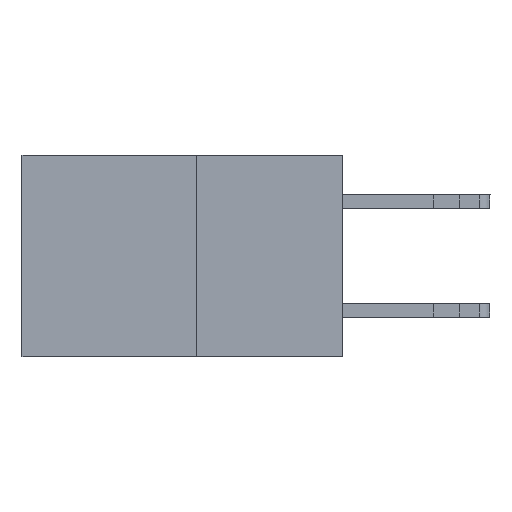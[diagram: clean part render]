
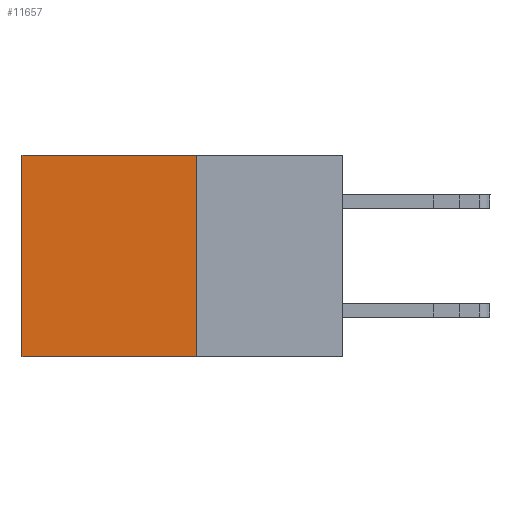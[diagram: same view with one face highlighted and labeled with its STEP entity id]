
A CAD part, left-side view. The second image highlights one B-rep face of the part: STEP entity #11657.
In plain terms, the highlighted planar face has unit normal (-1, 0, 0).
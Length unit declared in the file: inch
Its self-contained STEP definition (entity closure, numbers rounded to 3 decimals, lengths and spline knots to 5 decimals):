
#1325 = DIRECTION ( 'NONE',  ( 1., 0., 0. ) ) ;
#1469 = AXIS2_PLACEMENT_3D ( 'NONE', #7653, #1325, #16634 ) ;
#2169 = VECTOR ( 'NONE', #7233, 39.37008 ) ;
#3443 = CARTESIAN_POINT ( 'NONE',  ( 0.277, 0.27, 0. ) ) ;
#3674 = LINE ( 'NONE', #9184, #3949 ) ;
#3949 = VECTOR ( 'NONE', #5194, 39.37008 ) ;
#4091 = VECTOR ( 'NONE', #10835, 39.37008 ) ;
#5194 = DIRECTION ( 'NONE',  ( 0., 0., -1. ) ) ;
#5997 = CARTESIAN_POINT ( 'NONE',  ( 0.277, 0.59, -0.37 ) ) ;
#6428 = CARTESIAN_POINT ( 'NONE',  ( 0.277, 0.27, 0. ) ) ;
#7233 = DIRECTION ( 'NONE',  ( 0., 1., 0. ) ) ;
#7529 = PLANE ( 'NONE',  #1469 ) ;
#7653 = CARTESIAN_POINT ( 'NONE',  ( 0.277, 0.27, -0.37 ) ) ;
#7782 = FACE_OUTER_BOUND ( 'NONE', #18057, .T. ) ;
#9184 = CARTESIAN_POINT ( 'NONE',  ( 0.277, 0.59, -0.37 ) ) ;
#10682 = EDGE_CURVE ( 'NONE', #21772, #19550, #3674, .T. ) ;
#10835 = DIRECTION ( 'NONE',  ( 0., 1., 0. ) ) ;
#11657 = ADVANCED_FACE ( 'NONE', ( #7782 ), #7529, .F. ) ;
#13093 = ORIENTED_EDGE ( 'NONE', *, *, #20585, .F. ) ;
#15268 = VERTEX_POINT ( 'NONE', #6428 ) ;
#15631 = VECTOR ( 'NONE', #23907, 39.37008 ) ;
#15726 = CARTESIAN_POINT ( 'NONE',  ( 0.277, 0.59, 0. ) ) ;
#16035 = CARTESIAN_POINT ( 'NONE',  ( 0.277, 0.27, -0.37 ) ) ;
#16597 = ORIENTED_EDGE ( 'NONE', *, *, #10682, .T. ) ;
#16634 = DIRECTION ( 'NONE',  ( 0., 0., -1. ) ) ;
#17021 = LINE ( 'NONE', #24538, #2169 ) ;
#18057 = EDGE_LOOP ( 'NONE', ( #16597, #13093, #18802, #19836 ) ) ;
#18802 = ORIENTED_EDGE ( 'NONE', *, *, #23367, .F. ) ;
#19550 = VERTEX_POINT ( 'NONE', #5997 ) ;
#19741 = EDGE_CURVE ( 'NONE', #15268, #21772, #20612, .T. ) ;
#19836 = ORIENTED_EDGE ( 'NONE', *, *, #19741, .T. ) ;
#20003 = LINE ( 'NONE', #23535, #15631 ) ;
#20402 = VERTEX_POINT ( 'NONE', #16035 ) ;
#20585 = EDGE_CURVE ( 'NONE', #20402, #19550, #17021, .T. ) ;
#20612 = LINE ( 'NONE', #3443, #4091 ) ;
#21772 = VERTEX_POINT ( 'NONE', #15726 ) ;
#23367 = EDGE_CURVE ( 'NONE', #15268, #20402, #20003, .T. ) ;
#23535 = CARTESIAN_POINT ( 'NONE',  ( 0.277, 0.27, -0.37 ) ) ;
#23907 = DIRECTION ( 'NONE',  ( 0., 0., -1. ) ) ;
#24538 = CARTESIAN_POINT ( 'NONE',  ( 0.277, 0.27, -0.37 ) ) ;
